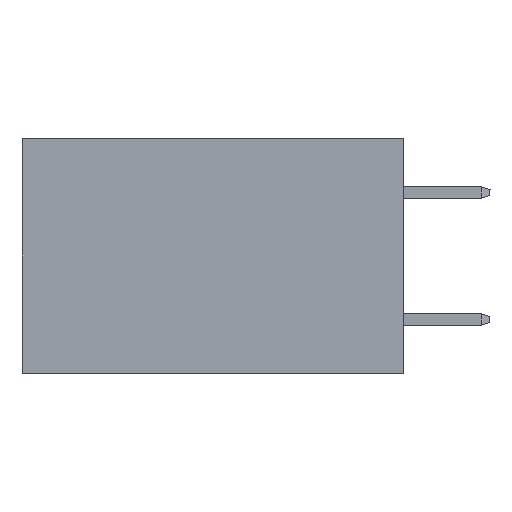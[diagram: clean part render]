
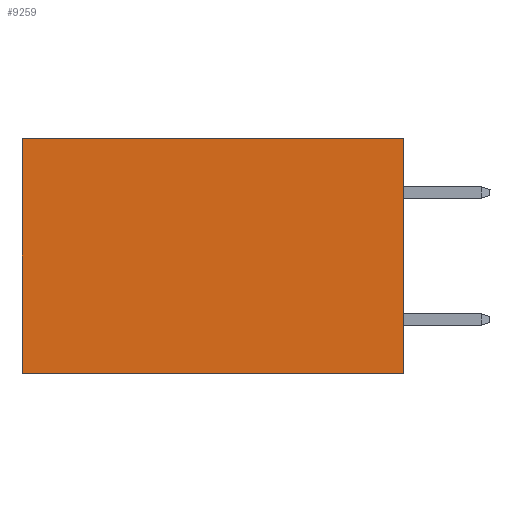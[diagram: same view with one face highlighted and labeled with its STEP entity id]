
A CAD part, left-side view. The second image highlights one B-rep face of the part: STEP entity #9259.
In plain terms, the highlighted planar face has unit normal (-1, 0, 0).
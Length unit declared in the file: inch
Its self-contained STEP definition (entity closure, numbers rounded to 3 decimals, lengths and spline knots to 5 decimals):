
#18 = DIRECTION ( 'NONE',  ( 0., 0., -1. ) ) ;
#1615 = VECTOR ( 'NONE', #2351, 39.37008 ) ;
#2351 = DIRECTION ( 'NONE',  ( 0., 0., -1. ) ) ;
#3835 = VERTEX_POINT ( 'NONE', #33026 ) ;
#3961 = DIRECTION ( 'NONE',  ( 0., 1., 0. ) ) ;
#5968 = CARTESIAN_POINT ( 'NONE',  ( 0.2875, 0., 0. ) ) ;
#6828 = DIRECTION ( 'NONE',  ( 0., 1., 0. ) ) ;
#8085 = CARTESIAN_POINT ( 'NONE',  ( 0.2875, 0.6, 0. ) ) ;
#9259 = ADVANCED_FACE ( 'NONE', ( #12443 ), #26907, .F. ) ;
#9599 = CARTESIAN_POINT ( 'NONE',  ( 0.2875, 0., 0. ) ) ;
#9796 = EDGE_CURVE ( 'NONE', #33824, #12458, #12596, .T. ) ;
#11146 = DIRECTION ( 'NONE',  ( 0., 0., -1. ) ) ;
#12068 = CARTESIAN_POINT ( 'NONE',  ( 0.2875, 0., 0. ) ) ;
#12443 = FACE_OUTER_BOUND ( 'NONE', #16021, .T. ) ;
#12458 = VERTEX_POINT ( 'NONE', #31665 ) ;
#12596 = LINE ( 'NONE', #24345, #35836 ) ;
#14691 = EDGE_CURVE ( 'NONE', #12458, #3835, #28693, .T. ) ;
#15530 = CARTESIAN_POINT ( 'NONE',  ( 0.2875, 0., -0.37 ) ) ;
#16021 = EDGE_LOOP ( 'NONE', ( #24232, #26276, #34477, #36579 ) ) ;
#18355 = CARTESIAN_POINT ( 'NONE',  ( 0.2875, 0., -0.37 ) ) ;
#18909 = VERTEX_POINT ( 'NONE', #15530 ) ;
#19814 = VECTOR ( 'NONE', #6828, 39.37008 ) ;
#24232 = ORIENTED_EDGE ( 'NONE', *, *, #14691, .T. ) ;
#24345 = CARTESIAN_POINT ( 'NONE',  ( 0.2875, 0., 0. ) ) ;
#26276 = ORIENTED_EDGE ( 'NONE', *, *, #36024, .F. ) ;
#26907 = PLANE ( 'NONE',  #34253 ) ;
#28693 = LINE ( 'NONE', #8085, #1615 ) ;
#29232 = DIRECTION ( 'NONE',  ( 1., 0., 0. ) ) ;
#30770 = VECTOR ( 'NONE', #11146, 39.37008 ) ;
#31665 = CARTESIAN_POINT ( 'NONE',  ( 0.2875, 0.6, 0. ) ) ;
#31964 = LINE ( 'NONE', #5968, #30770 ) ;
#32247 = EDGE_CURVE ( 'NONE', #33824, #18909, #31964, .T. ) ;
#33014 = LINE ( 'NONE', #18355, #19814 ) ;
#33026 = CARTESIAN_POINT ( 'NONE',  ( 0.2875, 0.6, -0.37 ) ) ;
#33824 = VERTEX_POINT ( 'NONE', #9599 ) ;
#34253 = AXIS2_PLACEMENT_3D ( 'NONE', #12068, #29232, #18 ) ;
#34477 = ORIENTED_EDGE ( 'NONE', *, *, #32247, .F. ) ;
#35836 = VECTOR ( 'NONE', #3961, 39.37008 ) ;
#36024 = EDGE_CURVE ( 'NONE', #18909, #3835, #33014, .T. ) ;
#36579 = ORIENTED_EDGE ( 'NONE', *, *, #9796, .T. ) ;
